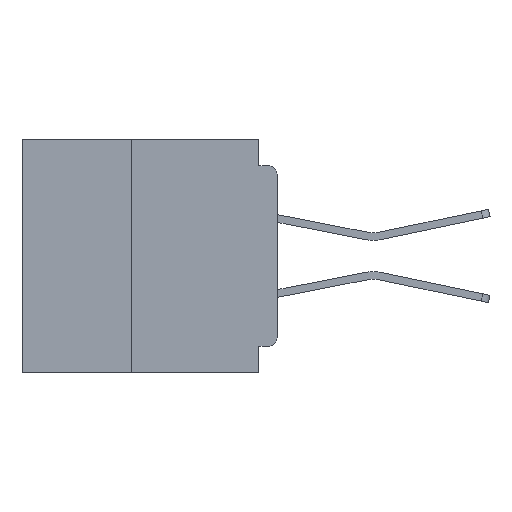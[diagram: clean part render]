
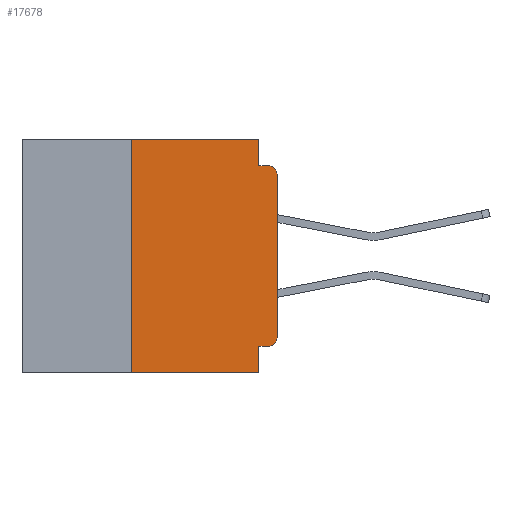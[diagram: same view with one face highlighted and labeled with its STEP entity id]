
A CAD part, left-side view. The second image highlights one B-rep face of the part: STEP entity #17678.
In plain terms, the highlighted planar face has unit normal (-1, 0, 0).
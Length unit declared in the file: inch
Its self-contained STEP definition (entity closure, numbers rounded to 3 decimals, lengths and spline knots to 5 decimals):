
#802 = ORIENTED_EDGE ( 'NONE', *, *, #55875, .F. ) ;
#966 = DIRECTION ( 'NONE',  ( 0., -1., 0. ) ) ;
#1373 = VERTEX_POINT ( 'NONE', #19918 ) ;
#1831 = CARTESIAN_POINT ( 'NONE',  ( 0., 0.031, 0. ) ) ;
#2248 = CARTESIAN_POINT ( 'NONE',  ( 0., 0., -0.045 ) ) ;
#2382 = ORIENTED_EDGE ( 'NONE', *, *, #11250, .F. ) ;
#3250 = LINE ( 'NONE', #27260, #4841 ) ;
#3742 = VERTEX_POINT ( 'NONE', #17367 ) ;
#4092 = PLANE ( 'NONE',  #44788 ) ;
#4841 = VECTOR ( 'NONE', #61685, 39.37008 ) ;
#6505 = CARTESIAN_POINT ( 'NONE',  ( 0., 0.25, -0.4 ) ) ;
#6858 = DIRECTION ( 'NONE',  ( 0., 0., -1. ) ) ;
#7178 = CARTESIAN_POINT ( 'NONE',  ( 0., 0.25, -0.4 ) ) ;
#7523 = CARTESIAN_POINT ( 'NONE',  ( 0., 0.015, -0.045 ) ) ;
#7889 = EDGE_LOOP ( 'NONE', ( #35172, #22134, #47869, #9511, #802, #10265, #40647, #2382, #29865, #39817 ) ) ;
#8673 = LINE ( 'NONE', #38007, #46453 ) ;
#9205 = VECTOR ( 'NONE', #41747, 39.37008 ) ;
#9511 = ORIENTED_EDGE ( 'NONE', *, *, #12287, .F. ) ;
#10265 = ORIENTED_EDGE ( 'NONE', *, *, #34836, .F. ) ;
#11250 = EDGE_CURVE ( 'NONE', #42944, #1373, #3250, .T. ) ;
#11368 = EDGE_CURVE ( 'NONE', #23794, #42944, #8673, .T. ) ;
#12128 = DIRECTION ( 'NONE',  ( 0., 0., 1. ) ) ;
#12287 = EDGE_CURVE ( 'NONE', #24939, #45962, #44795, .T. ) ;
#14017 = CARTESIAN_POINT ( 'NONE',  ( 0., 0.437, 0. ) ) ;
#15839 = CARTESIAN_POINT ( 'NONE',  ( 0., 0.25, 0. ) ) ;
#17367 = CARTESIAN_POINT ( 'NONE',  ( 0., 0., -0.34 ) ) ;
#17674 = CARTESIAN_POINT ( 'NONE',  ( 0., 0.015, -0.355 ) ) ;
#17678 = ADVANCED_FACE ( 'NONE', ( #33761 ), #4092, .F. ) ;
#18569 = VECTOR ( 'NONE', #6858, 39.37008 ) ;
#19382 = VERTEX_POINT ( 'NONE', #15839 ) ;
#19918 = CARTESIAN_POINT ( 'NONE',  ( 0., 0.031, -0.4 ) ) ;
#22134 = ORIENTED_EDGE ( 'NONE', *, *, #45181, .T. ) ;
#22350 = VECTOR ( 'NONE', #966, 39.37008 ) ;
#23726 = VECTOR ( 'NONE', #44970, 39.37008 ) ;
#23794 = VERTEX_POINT ( 'NONE', #17674 ) ;
#23946 = DIRECTION ( 'NONE',  ( 1., 0., 0. ) ) ;
#24179 = EDGE_CURVE ( 'NONE', #62926, #1373, #35530, .T. ) ;
#24846 = DIRECTION ( 'NONE',  ( -1., 0., 0. ) ) ;
#24939 = VERTEX_POINT ( 'NONE', #33955 ) ;
#25215 = AXIS2_PLACEMENT_3D ( 'NONE', #26829, #61254, #31823 ) ;
#26829 = CARTESIAN_POINT ( 'NONE',  ( 0., 0.015, -0.06 ) ) ;
#27260 = CARTESIAN_POINT ( 'NONE',  ( 0., 0.031, -0.4 ) ) ;
#28494 = CIRCLE ( 'NONE', #25215, 0.015 ) ;
#29865 = ORIENTED_EDGE ( 'NONE', *, *, #11368, .F. ) ;
#30481 = LINE ( 'NONE', #32108, #56651 ) ;
#30516 = AXIS2_PLACEMENT_3D ( 'NONE', #54359, #24846, #59346 ) ;
#31823 = DIRECTION ( 'NONE',  ( 0., 0., -1. ) ) ;
#32108 = CARTESIAN_POINT ( 'NONE',  ( 0., 0., 0. ) ) ;
#33761 = FACE_OUTER_BOUND ( 'NONE', #7889, .T. ) ;
#33932 = LINE ( 'NONE', #2248, #9205 ) ;
#33955 = CARTESIAN_POINT ( 'NONE',  ( 0., 0.031, 0. ) ) ;
#34107 = VERTEX_POINT ( 'NONE', #55771 ) ;
#34836 = EDGE_CURVE ( 'NONE', #62926, #19382, #53242, .T. ) ;
#35134 = CIRCLE ( 'NONE', #30516, 0.015 ) ;
#35172 = ORIENTED_EDGE ( 'NONE', *, *, #36077, .T. ) ;
#35530 = LINE ( 'NONE', #50165, #22350 ) ;
#36077 = EDGE_CURVE ( 'NONE', #3742, #34107, #30481, .T. ) ;
#37701 = CARTESIAN_POINT ( 'NONE',  ( 0., 0.031, -0.355 ) ) ;
#38007 = CARTESIAN_POINT ( 'NONE',  ( 0., 0., -0.355 ) ) ;
#39817 = ORIENTED_EDGE ( 'NONE', *, *, #62749, .T. ) ;
#40058 = CARTESIAN_POINT ( 'NONE',  ( 0., 0.437, 0. ) ) ;
#40171 = VECTOR ( 'NONE', #12128, 39.37008 ) ;
#40647 = ORIENTED_EDGE ( 'NONE', *, *, #24179, .T. ) ;
#41747 = DIRECTION ( 'NONE',  ( 0., -1., 0. ) ) ;
#42944 = VERTEX_POINT ( 'NONE', #37701 ) ;
#44788 = AXIS2_PLACEMENT_3D ( 'NONE', #14017, #23946, #58444 ) ;
#44795 = LINE ( 'NONE', #1831, #18569 ) ;
#44970 = DIRECTION ( 'NONE',  ( 0., -1., 0. ) ) ;
#45181 = EDGE_CURVE ( 'NONE', #34107, #58634, #28494, .T. ) ;
#45962 = VERTEX_POINT ( 'NONE', #57333 ) ;
#46453 = VECTOR ( 'NONE', #52846, 39.37008 ) ;
#47869 = ORIENTED_EDGE ( 'NONE', *, *, #60220, .F. ) ;
#50165 = CARTESIAN_POINT ( 'NONE',  ( 0., 0.437, -0.4 ) ) ;
#52846 = DIRECTION ( 'NONE',  ( 0., 1., 0. ) ) ;
#53242 = LINE ( 'NONE', #7178, #40171 ) ;
#54359 = CARTESIAN_POINT ( 'NONE',  ( 0., 0.015, -0.34 ) ) ;
#55771 = CARTESIAN_POINT ( 'NONE',  ( 0., 0., -0.06 ) ) ;
#55875 = EDGE_CURVE ( 'NONE', #19382, #24939, #63015, .T. ) ;
#56651 = VECTOR ( 'NONE', #56950, 39.37008 ) ;
#56950 = DIRECTION ( 'NONE',  ( 0., 0., 1. ) ) ;
#57333 = CARTESIAN_POINT ( 'NONE',  ( 0., 0.031, -0.045 ) ) ;
#58444 = DIRECTION ( 'NONE',  ( 0., 0., -1. ) ) ;
#58634 = VERTEX_POINT ( 'NONE', #7523 ) ;
#59346 = DIRECTION ( 'NONE',  ( 0., 0., -1. ) ) ;
#60220 = EDGE_CURVE ( 'NONE', #45962, #58634, #33932, .T. ) ;
#61254 = DIRECTION ( 'NONE',  ( -1., 0., 0. ) ) ;
#61685 = DIRECTION ( 'NONE',  ( 0., 0., -1. ) ) ;
#62749 = EDGE_CURVE ( 'NONE', #23794, #3742, #35134, .T. ) ;
#62926 = VERTEX_POINT ( 'NONE', #6505 ) ;
#63015 = LINE ( 'NONE', #40058, #23726 ) ;
